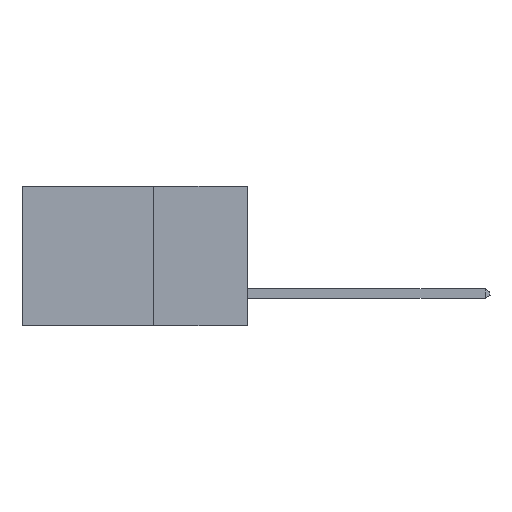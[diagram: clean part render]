
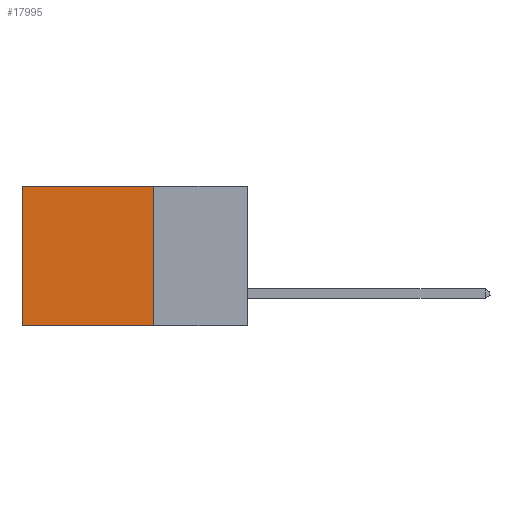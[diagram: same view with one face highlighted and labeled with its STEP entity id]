
A CAD part, left-side view. The second image highlights one B-rep face of the part: STEP entity #17995.
In plain terms, the highlighted planar face has unit normal (-1, 0, 0).
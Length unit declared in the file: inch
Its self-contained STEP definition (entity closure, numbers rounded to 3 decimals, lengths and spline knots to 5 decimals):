
#260 = VERTEX_POINT ( 'NONE', #7434 ) ;
#803 = AXIS2_PLACEMENT_3D ( 'NONE', #3190, #12673, #18449 ) ;
#873 = ORIENTED_EDGE ( 'NONE', *, *, #2475, .F. ) ;
#1735 = LINE ( 'NONE', #22299, #20333 ) ;
#1787 = DIRECTION ( 'NONE',  ( 0., 0., -1. ) ) ;
#1876 = CARTESIAN_POINT ( 'NONE',  ( 0.298, 0.6, 0. ) ) ;
#2336 = ORIENTED_EDGE ( 'NONE', *, *, #15708, .T. ) ;
#2475 = EDGE_CURVE ( 'NONE', #260, #15689, #18400, .T. ) ;
#3042 = VERTEX_POINT ( 'NONE', #23266 ) ;
#3190 = CARTESIAN_POINT ( 'NONE',  ( 0.298, 0.25, 0. ) ) ;
#3705 = VECTOR ( 'NONE', #12910, 39.37008 ) ;
#4236 = CARTESIAN_POINT ( 'NONE',  ( 0.298, 0.25, 0. ) ) ;
#5984 = CARTESIAN_POINT ( 'NONE',  ( 0.298, 0.6, 0. ) ) ;
#7028 = DIRECTION ( 'NONE',  ( 0., 1., 0. ) ) ;
#7063 = ORIENTED_EDGE ( 'NONE', *, *, #15532, .T. ) ;
#7434 = CARTESIAN_POINT ( 'NONE',  ( 0.298, 0.25, 0. ) ) ;
#7535 = LINE ( 'NONE', #4236, #21996 ) ;
#8659 = VECTOR ( 'NONE', #1787, 39.37008 ) ;
#10502 = FACE_OUTER_BOUND ( 'NONE', #24380, .T. ) ;
#11034 = EDGE_CURVE ( 'NONE', #15689, #3042, #1735, .T. ) ;
#12673 = DIRECTION ( 'NONE',  ( 1., 0., 0. ) ) ;
#12910 = DIRECTION ( 'NONE',  ( 0., 0., -1. ) ) ;
#15203 = LINE ( 'NONE', #1876, #3705 ) ;
#15532 = EDGE_CURVE ( 'NONE', #18423, #3042, #15203, .T. ) ;
#15689 = VERTEX_POINT ( 'NONE', #17919 ) ;
#15708 = EDGE_CURVE ( 'NONE', #260, #18423, #7535, .T. ) ;
#16669 = DIRECTION ( 'NONE',  ( 0., 1., 0. ) ) ;
#16961 = CARTESIAN_POINT ( 'NONE',  ( 0.298, 0.25, 0. ) ) ;
#17919 = CARTESIAN_POINT ( 'NONE',  ( 0.298, 0.25, -0.37 ) ) ;
#17995 = ADVANCED_FACE ( 'NONE', ( #10502 ), #23998, .F. ) ;
#18400 = LINE ( 'NONE', #16961, #8659 ) ;
#18423 = VERTEX_POINT ( 'NONE', #5984 ) ;
#18449 = DIRECTION ( 'NONE',  ( 0., 0., -1. ) ) ;
#18578 = ORIENTED_EDGE ( 'NONE', *, *, #11034, .F. ) ;
#20333 = VECTOR ( 'NONE', #16669, 39.37008 ) ;
#21996 = VECTOR ( 'NONE', #7028, 39.37008 ) ;
#22299 = CARTESIAN_POINT ( 'NONE',  ( 0.298, 0.25, -0.37 ) ) ;
#23266 = CARTESIAN_POINT ( 'NONE',  ( 0.298, 0.6, -0.37 ) ) ;
#23998 = PLANE ( 'NONE',  #803 ) ;
#24380 = EDGE_LOOP ( 'NONE', ( #7063, #18578, #873, #2336 ) ) ;
